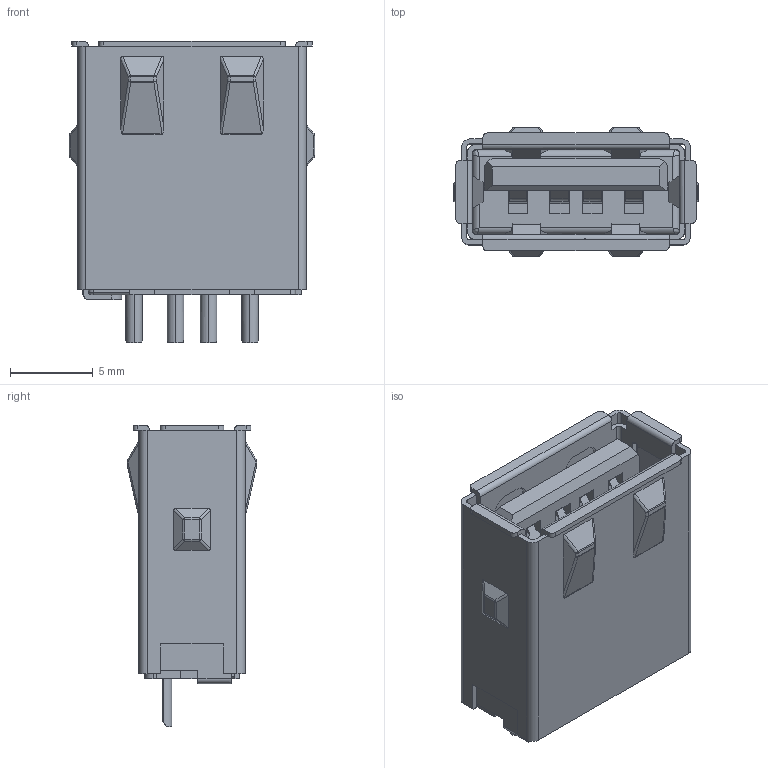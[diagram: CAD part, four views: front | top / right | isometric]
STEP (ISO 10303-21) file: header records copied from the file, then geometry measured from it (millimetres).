
FILE_DESCRIPTION (( 'STEP AP214' ), '1' );
FILE_NAME ('690L104J19D-020.STEP', '2021-01-14T14:10:54', ( '' ), ( '' ), 'SwSTEP 2.0', 'SolidWorks 2020', '' );
FILE_SCHEMA (( 'AUTOMOTIVE_DESIGN' ));
Length unit declared in the file: millimetre
Products named in the file (6): Contact 690L104JX9D-02X; Shell 690L104JX9D-02X; Insulator 2 690L104JX9D-02X_White; 690L104J19D-020; Jacket 690L104JX9D-02X; Insulator 690L104JX9D-02X_White
Assembly tree (8 placements, depth 2):
  690L104J19D-020
    Insulator 690L104JX9D-02X_White
    Contact 690L104JX9D-02X  x4
    Insulator 2 690L104JX9D-02X_White
    Shell 690L104JX9D-02X
    Jacket 690L104JX9D-02X
Bounding box: 14.8 x 7.8 x 18.2 mm (x, y, z)
Volume: 792.7 mm3; surface area: 3425.2 mm2
Topology: 8 solids, 8 shells, 1045 faces, 2971 edges, 1903 vertices
Faces by surface type: plane 678, cylinder 297, bspline 70
Entity records: 30395 total; most frequent: CARTESIAN_POINT 8925, ORIENTED_EDGE 4798, DIRECTION 3878, EDGE_CURVE 2399, LINE 1766, VECTOR 1766, VERTEX_POINT 1555, AXIS2_PLACEMENT_3D 1056
